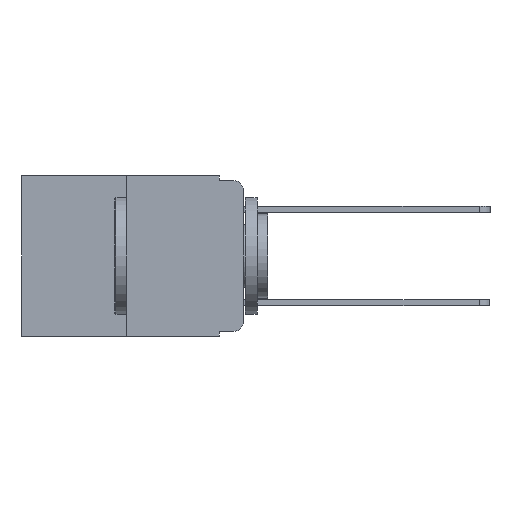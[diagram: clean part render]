
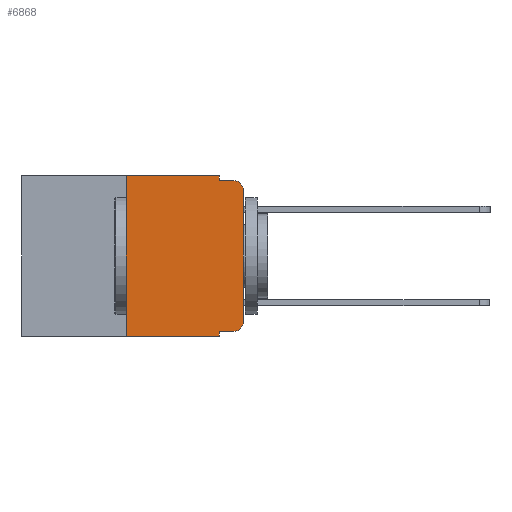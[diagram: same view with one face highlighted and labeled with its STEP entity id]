
A CAD part, left-side view. The second image highlights one B-rep face of the part: STEP entity #6868.
In plain terms, the highlighted planar face has unit normal (-1, 0, 0).
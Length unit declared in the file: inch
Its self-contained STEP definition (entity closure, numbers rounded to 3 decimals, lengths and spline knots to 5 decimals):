
#228 = EDGE_CURVE ( 'NONE', #12268, #7184, #8787, .T. ) ;
#329 = EDGE_CURVE ( 'NONE', #1222, #12268, #9243, .T. ) ;
#606 = VERTEX_POINT ( 'NONE', #2285 ) ;
#724 = DIRECTION ( 'NONE',  ( 0., -1., 0. ) ) ;
#732 = LINE ( 'NONE', #4101, #8990 ) ;
#775 = CIRCLE ( 'NONE', #13153, 0.02 ) ;
#1148 = EDGE_CURVE ( 'NONE', #7184, #8004, #12918, .T. ) ;
#1222 = VERTEX_POINT ( 'NONE', #11331 ) ;
#1368 = DIRECTION ( 'NONE',  ( 0., 0., -1. ) ) ;
#1379 = DIRECTION ( 'NONE',  ( 0., 0., 1. ) ) ;
#1779 = CARTESIAN_POINT ( 'NONE',  ( 0., 0.051, -0.333 ) ) ;
#1852 = ORIENTED_EDGE ( 'NONE', *, *, #329, .F. ) ;
#2011 = EDGE_CURVE ( 'NONE', #8004, #7363, #732, .T. ) ;
#2285 = CARTESIAN_POINT ( 'NONE',  ( 0., 0., -0.313 ) ) ;
#2405 = DIRECTION ( 'NONE',  ( 0., -1., 0. ) ) ;
#2436 = CARTESIAN_POINT ( 'NONE',  ( 0., 0.02, -0.01 ) ) ;
#2763 = EDGE_CURVE ( 'NONE', #4258, #7363, #5775, .T. ) ;
#2872 = DIRECTION ( 'NONE',  ( 0., 0., -1. ) ) ;
#3002 = LINE ( 'NONE', #10047, #5464 ) ;
#3285 = VECTOR ( 'NONE', #724, 39.37008 ) ;
#3346 = DIRECTION ( 'NONE',  ( 0., 0., 1. ) ) ;
#3499 = EDGE_CURVE ( 'NONE', #606, #4258, #9402, .T. ) ;
#3933 = VECTOR ( 'NONE', #1379, 39.37008 ) ;
#3979 = DIRECTION ( 'NONE',  ( 0., -1., 0. ) ) ;
#4101 = CARTESIAN_POINT ( 'NONE',  ( 0., 0.051, -0.01 ) ) ;
#4177 = CARTESIAN_POINT ( 'NONE',  ( 0., 0.02, -0.313 ) ) ;
#4258 = VERTEX_POINT ( 'NONE', #12736 ) ;
#4647 = EDGE_CURVE ( 'NONE', #1222, #5745, #7493, .T. ) ;
#4725 = CARTESIAN_POINT ( 'NONE',  ( 0., 0.25, 0. ) ) ;
#5220 = DIRECTION ( 'NONE',  ( 0., 0., -1. ) ) ;
#5372 = VECTOR ( 'NONE', #12489, 39.37008 ) ;
#5388 = CARTESIAN_POINT ( 'NONE',  ( 0., 0.051, -0.343 ) ) ;
#5397 = CARTESIAN_POINT ( 'NONE',  ( 0., 0.051, 0. ) ) ;
#5452 = VECTOR ( 'NONE', #1368, 39.37008 ) ;
#5464 = VECTOR ( 'NONE', #3979, 39.37008 ) ;
#5545 = CARTESIAN_POINT ( 'NONE',  ( 0., 0.473, -0.343 ) ) ;
#5745 = VERTEX_POINT ( 'NONE', #5388 ) ;
#5775 = CIRCLE ( 'NONE', #7917, 0.02 ) ;
#5805 = EDGE_LOOP ( 'NONE', ( #7995, #5906, #11246, #6573, #12109, #1852, #11105, #8781, #11392, #11970 ) ) ;
#5906 = ORIENTED_EDGE ( 'NONE', *, *, #2763, .T. ) ;
#6018 = CARTESIAN_POINT ( 'NONE',  ( 0., 0.473, 0. ) ) ;
#6239 = VERTEX_POINT ( 'NONE', #1779 ) ;
#6573 = ORIENTED_EDGE ( 'NONE', *, *, #1148, .F. ) ;
#6581 = VECTOR ( 'NONE', #3346, 39.37008 ) ;
#6610 = CARTESIAN_POINT ( 'NONE',  ( 0., 0.473, 0. ) ) ;
#6832 = CARTESIAN_POINT ( 'NONE',  ( 0., 0.051, 0. ) ) ;
#6868 = ADVANCED_FACE ( 'NONE', ( #12899 ), #12887, .F. ) ;
#7006 = DIRECTION ( 'NONE',  ( 0., 0., -1. ) ) ;
#7044 = DIRECTION ( 'NONE',  ( -1., 0., 0. ) ) ;
#7055 = CARTESIAN_POINT ( 'NONE',  ( 0., 0.02, -0.03 ) ) ;
#7184 = VERTEX_POINT ( 'NONE', #13276 ) ;
#7363 = VERTEX_POINT ( 'NONE', #2436 ) ;
#7493 = LINE ( 'NONE', #5545, #5372 ) ;
#7888 = LINE ( 'NONE', #6832, #5452 ) ;
#7917 = AXIS2_PLACEMENT_3D ( 'NONE', #7055, #7044, #8705 ) ;
#7959 = AXIS2_PLACEMENT_3D ( 'NONE', #6018, #9086, #2872 ) ;
#7995 = ORIENTED_EDGE ( 'NONE', *, *, #3499, .T. ) ;
#8004 = VERTEX_POINT ( 'NONE', #8584 ) ;
#8584 = CARTESIAN_POINT ( 'NONE',  ( 0., 0.051, -0.01 ) ) ;
#8705 = DIRECTION ( 'NONE',  ( 0., 0., -1. ) ) ;
#8781 = ORIENTED_EDGE ( 'NONE', *, *, #13098, .F. ) ;
#8787 = LINE ( 'NONE', #6610, #3285 ) ;
#8990 = VECTOR ( 'NONE', #2405, 39.37008 ) ;
#9086 = DIRECTION ( 'NONE',  ( 1., 0., 0. ) ) ;
#9243 = LINE ( 'NONE', #13343, #6581 ) ;
#9402 = LINE ( 'NONE', #12667, #3933 ) ;
#10047 = CARTESIAN_POINT ( 'NONE',  ( 0., 0.051, -0.333 ) ) ;
#10427 = VECTOR ( 'NONE', #7006, 39.37008 ) ;
#11105 = ORIENTED_EDGE ( 'NONE', *, *, #4647, .T. ) ;
#11246 = ORIENTED_EDGE ( 'NONE', *, *, #2011, .F. ) ;
#11276 = DIRECTION ( 'NONE',  ( -1., 0., 0. ) ) ;
#11331 = CARTESIAN_POINT ( 'NONE',  ( 0., 0.25, -0.343 ) ) ;
#11392 = ORIENTED_EDGE ( 'NONE', *, *, #12496, .T. ) ;
#11867 = EDGE_CURVE ( 'NONE', #12704, #606, #775, .T. ) ;
#11970 = ORIENTED_EDGE ( 'NONE', *, *, #11867, .T. ) ;
#12109 = ORIENTED_EDGE ( 'NONE', *, *, #228, .F. ) ;
#12268 = VERTEX_POINT ( 'NONE', #4725 ) ;
#12489 = DIRECTION ( 'NONE',  ( 0., -1., 0. ) ) ;
#12496 = EDGE_CURVE ( 'NONE', #6239, #12704, #3002, .T. ) ;
#12667 = CARTESIAN_POINT ( 'NONE',  ( 0., 0., 0. ) ) ;
#12704 = VERTEX_POINT ( 'NONE', #13144 ) ;
#12736 = CARTESIAN_POINT ( 'NONE',  ( 0., 0., -0.03 ) ) ;
#12887 = PLANE ( 'NONE',  #7959 ) ;
#12899 = FACE_OUTER_BOUND ( 'NONE', #5805, .T. ) ;
#12918 = LINE ( 'NONE', #5397, #10427 ) ;
#13098 = EDGE_CURVE ( 'NONE', #6239, #5745, #7888, .T. ) ;
#13144 = CARTESIAN_POINT ( 'NONE',  ( 0., 0.02, -0.333 ) ) ;
#13153 = AXIS2_PLACEMENT_3D ( 'NONE', #4177, #11276, #5220 ) ;
#13276 = CARTESIAN_POINT ( 'NONE',  ( 0., 0.051, 0. ) ) ;
#13343 = CARTESIAN_POINT ( 'NONE',  ( 0., 0.25, 0. ) ) ;
